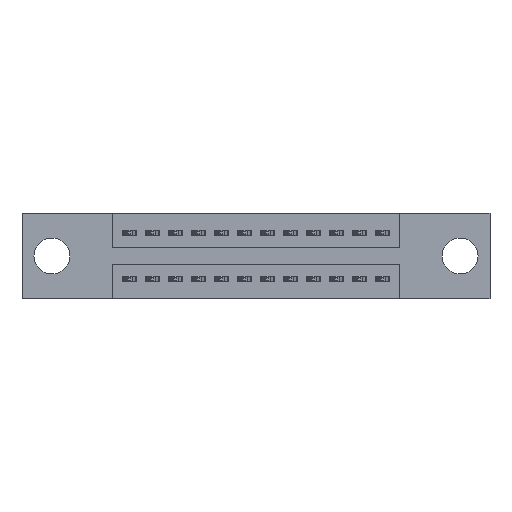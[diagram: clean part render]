
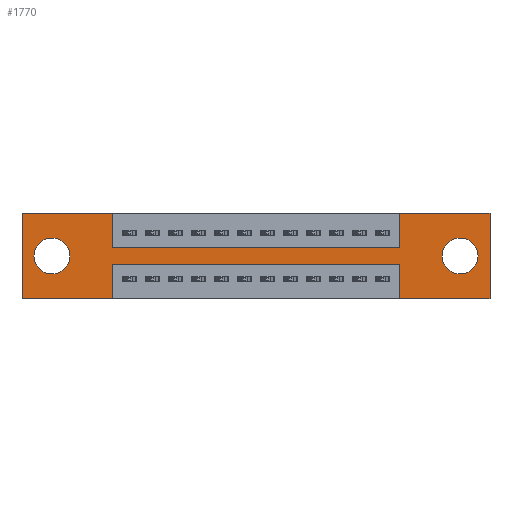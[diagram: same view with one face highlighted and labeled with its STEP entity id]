
A CAD part, front view. The second image highlights one B-rep face of the part: STEP entity #1770.
In plain terms, the highlighted planar face has unit normal (0, -1, 0).
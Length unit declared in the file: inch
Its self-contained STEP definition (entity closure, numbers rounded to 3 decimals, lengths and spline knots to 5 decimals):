
#2 = DIRECTION ( 'NONE',  ( 0., 0., -1. ) ) ;
#174 = DIRECTION ( 'NONE',  ( 0., -1., 0. ) ) ;
#203 = DIRECTION ( 'NONE',  ( 0., 0., -1. ) ) ;
#253 = CARTESIAN_POINT ( 'NONE',  ( 1.905, 0., -0.185 ) ) ;
#275 = LINE ( 'NONE', #10643, #8796 ) ;
#563 = DIRECTION ( 'NONE',  ( 0., 0., -1. ) ) ;
#569 = DIRECTION ( 'NONE',  ( 1., 0., 0. ) ) ;
#719 = VERTEX_POINT ( 'NONE', #10996 ) ;
#798 = CIRCLE ( 'NONE', #2338, 0.078 ) ;
#893 = EDGE_CURVE ( 'NONE', #12696, #719, #12292, .T. ) ;
#922 = VECTOR ( 'NONE', #13140, 39.37008 ) ;
#1003 = ORIENTED_EDGE ( 'NONE', *, *, #2645, .F. ) ;
#1030 = ORIENTED_EDGE ( 'NONE', *, *, #3036, .F. ) ;
#1304 = EDGE_CURVE ( 'NONE', #5290, #9071, #12277, .T. ) ;
#1329 = EDGE_LOOP ( 'NONE', ( #4029, #4434 ) ) ;
#1459 = DIRECTION ( 'NONE',  ( 0., 0., -1. ) ) ;
#1677 = CARTESIAN_POINT ( 'NONE',  ( 0., 0., -0.37 ) ) ;
#1770 = ADVANCED_FACE ( 'NONE', ( #9469, #12102, #7418 ), #4141, .T. ) ;
#1954 = DIRECTION ( 'NONE',  ( 1., 0., 0. ) ) ;
#2064 = ORIENTED_EDGE ( 'NONE', *, *, #10135, .F. ) ;
#2110 = CARTESIAN_POINT ( 'NONE',  ( 0.13, 0., -0.263 ) ) ;
#2338 = AXIS2_PLACEMENT_3D ( 'NONE', #253, #7798, #1459 ) ;
#2645 = EDGE_CURVE ( 'NONE', #11513, #3773, #12827, .T. ) ;
#2781 = LINE ( 'NONE', #10382, #10631 ) ;
#2795 = VECTOR ( 'NONE', #8695, 39.37008 ) ;
#2805 = VERTEX_POINT ( 'NONE', #12296 ) ;
#2915 = VECTOR ( 'NONE', #6998, 39.37008 ) ;
#3036 = EDGE_CURVE ( 'NONE', #3773, #12247, #275, .T. ) ;
#3151 = CARTESIAN_POINT ( 'NONE',  ( 0.3925, 0., -0.15 ) ) ;
#3304 = LINE ( 'NONE', #12684, #8466 ) ;
#3378 = ORIENTED_EDGE ( 'NONE', *, *, #8499, .T. ) ;
#3497 = CARTESIAN_POINT ( 'NONE',  ( 2.035, 0., 0. ) ) ;
#3583 = AXIS2_PLACEMENT_3D ( 'NONE', #12540, #6571, #2 ) ;
#3650 = ORIENTED_EDGE ( 'NONE', *, *, #12038, .F. ) ;
#3750 = VERTEX_POINT ( 'NONE', #4860 ) ;
#3773 = VERTEX_POINT ( 'NONE', #4777 ) ;
#3860 = ORIENTED_EDGE ( 'NONE', *, *, #7629, .T. ) ;
#3925 = EDGE_LOOP ( 'NONE', ( #6591, #10969, #7562, #7850, #9194, #2064, #1030, #1003, #3650, #5429, #10822, #8170 ) ) ;
#4004 = CARTESIAN_POINT ( 'NONE',  ( 2.035, 0., 0. ) ) ;
#4029 = ORIENTED_EDGE ( 'NONE', *, *, #4205, .T. ) ;
#4141 = PLANE ( 'NONE',  #5657 ) ;
#4205 = EDGE_CURVE ( 'NONE', #9071, #5290, #13422, .T. ) ;
#4434 = ORIENTED_EDGE ( 'NONE', *, *, #1304, .T. ) ;
#4455 = CARTESIAN_POINT ( 'NONE',  ( 0.3925, 0., -0.22 ) ) ;
#4621 = EDGE_CURVE ( 'NONE', #719, #4875, #3304, .T. ) ;
#4636 = VERTEX_POINT ( 'NONE', #11166 ) ;
#4777 = CARTESIAN_POINT ( 'NONE',  ( 1.6425, 0., -0.15 ) ) ;
#4835 = DIRECTION ( 'NONE',  ( 0., 1., 0. ) ) ;
#4860 = CARTESIAN_POINT ( 'NONE',  ( 0., 0., -0.37 ) ) ;
#4875 = VERTEX_POINT ( 'NONE', #5121 ) ;
#5099 = CARTESIAN_POINT ( 'NONE',  ( 1.905, 0., -0.263 ) ) ;
#5121 = CARTESIAN_POINT ( 'NONE',  ( 1.6425, 0., -0.22 ) ) ;
#5290 = VERTEX_POINT ( 'NONE', #2110 ) ;
#5429 = ORIENTED_EDGE ( 'NONE', *, *, #13178, .F. ) ;
#5558 = VECTOR ( 'NONE', #6076, 39.37008 ) ;
#5657 = AXIS2_PLACEMENT_3D ( 'NONE', #11202, #174, #203 ) ;
#5718 = LINE ( 'NONE', #11992, #2915 ) ;
#5762 = VERTEX_POINT ( 'NONE', #5099 ) ;
#5989 = DIRECTION ( 'NONE',  ( -1., 0., 0. ) ) ;
#6076 = DIRECTION ( 'NONE',  ( 0., 0., -1. ) ) ;
#6476 = CARTESIAN_POINT ( 'NONE',  ( 2.035, 0., -0.37 ) ) ;
#6571 = DIRECTION ( 'NONE',  ( 0., 1., 0. ) ) ;
#6591 = ORIENTED_EDGE ( 'NONE', *, *, #11502, .F. ) ;
#6746 = EDGE_LOOP ( 'NONE', ( #3378, #3860 ) ) ;
#6996 = VECTOR ( 'NONE', #569, 39.37008 ) ;
#6998 = DIRECTION ( 'NONE',  ( 1., 0., 0. ) ) ;
#7048 = DIRECTION ( 'NONE',  ( 0., 0., 1. ) ) ;
#7371 = AXIS2_PLACEMENT_3D ( 'NONE', #11588, #10906, #10991 ) ;
#7418 = FACE_OUTER_BOUND ( 'NONE', #3925, .T. ) ;
#7511 = CARTESIAN_POINT ( 'NONE',  ( 0.13, 0., -0.107 ) ) ;
#7540 = VECTOR ( 'NONE', #1954, 39.37008 ) ;
#7562 = ORIENTED_EDGE ( 'NONE', *, *, #4621, .F. ) ;
#7629 = EDGE_CURVE ( 'NONE', #5762, #2805, #8946, .T. ) ;
#7676 = CARTESIAN_POINT ( 'NONE',  ( 0.3925, 0., 0. ) ) ;
#7798 = DIRECTION ( 'NONE',  ( 0., 1., 0. ) ) ;
#7807 = VERTEX_POINT ( 'NONE', #9737 ) ;
#7850 = ORIENTED_EDGE ( 'NONE', *, *, #893, .F. ) ;
#7951 = EDGE_CURVE ( 'NONE', #7807, #3750, #12496, .T. ) ;
#8170 = ORIENTED_EDGE ( 'NONE', *, *, #7951, .F. ) ;
#8466 = VECTOR ( 'NONE', #11372, 39.37008 ) ;
#8499 = EDGE_CURVE ( 'NONE', #2805, #5762, #798, .T. ) ;
#8695 = DIRECTION ( 'NONE',  ( 0., 0., -1. ) ) ;
#8796 = VECTOR ( 'NONE', #10608, 39.37008 ) ;
#8946 = CIRCLE ( 'NONE', #3583, 0.078 ) ;
#9071 = VERTEX_POINT ( 'NONE', #7511 ) ;
#9084 = EDGE_CURVE ( 'NONE', #4875, #12977, #12925, .T. ) ;
#9194 = ORIENTED_EDGE ( 'NONE', *, *, #10892, .F. ) ;
#9469 = FACE_BOUND ( 'NONE', #6746, .T. ) ;
#9737 = CARTESIAN_POINT ( 'NONE',  ( 0.3925, 0., -0.37 ) ) ;
#9957 = CARTESIAN_POINT ( 'NONE',  ( 1.6425, 0., 0. ) ) ;
#10007 = VECTOR ( 'NONE', #12520, 39.37008 ) ;
#10034 = AXIS2_PLACEMENT_3D ( 'NONE', #10175, #4835, #7048 ) ;
#10135 = EDGE_CURVE ( 'NONE', #12247, #12814, #5718, .T. ) ;
#10154 = CARTESIAN_POINT ( 'NONE',  ( 0., 0., -0.37 ) ) ;
#10175 = CARTESIAN_POINT ( 'NONE',  ( 0.13, 0., -0.185 ) ) ;
#10382 = CARTESIAN_POINT ( 'NONE',  ( 0., 0., 0. ) ) ;
#10608 = DIRECTION ( 'NONE',  ( 0., 0., 1. ) ) ;
#10631 = VECTOR ( 'NONE', #11397, 39.37008 ) ;
#10643 = CARTESIAN_POINT ( 'NONE',  ( 1.6425, 0., 0. ) ) ;
#10661 = VERTEX_POINT ( 'NONE', #12783 ) ;
#10822 = ORIENTED_EDGE ( 'NONE', *, *, #12610, .F. ) ;
#10891 = LINE ( 'NONE', #4004, #5558 ) ;
#10892 = EDGE_CURVE ( 'NONE', #12814, #12696, #10891, .T. ) ;
#10906 = DIRECTION ( 'NONE',  ( 0., 1., 0. ) ) ;
#10959 = LINE ( 'NONE', #7676, #2795 ) ;
#10969 = ORIENTED_EDGE ( 'NONE', *, *, #9084, .F. ) ;
#10991 = DIRECTION ( 'NONE',  ( 0., 0., 1. ) ) ;
#10996 = CARTESIAN_POINT ( 'NONE',  ( 1.6425, 0., -0.37 ) ) ;
#11166 = CARTESIAN_POINT ( 'NONE',  ( 0., 0., 0. ) ) ;
#11202 = CARTESIAN_POINT ( 'NONE',  ( 0., 0., -0.37 ) ) ;
#11292 = VECTOR ( 'NONE', #563, 39.37008 ) ;
#11372 = DIRECTION ( 'NONE',  ( 0., 0., 1. ) ) ;
#11397 = DIRECTION ( 'NONE',  ( 0., 0., 1. ) ) ;
#11502 = EDGE_CURVE ( 'NONE', #12977, #7807, #11597, .T. ) ;
#11513 = VERTEX_POINT ( 'NONE', #12044 ) ;
#11588 = CARTESIAN_POINT ( 'NONE',  ( 0.13, 0., -0.185 ) ) ;
#11597 = LINE ( 'NONE', #12981, #11292 ) ;
#11847 = CARTESIAN_POINT ( 'NONE',  ( 0.3925, 0., -0.22 ) ) ;
#11992 = CARTESIAN_POINT ( 'NONE',  ( 0., 0., 0. ) ) ;
#12038 = EDGE_CURVE ( 'NONE', #10661, #11513, #10959, .T. ) ;
#12044 = CARTESIAN_POINT ( 'NONE',  ( 0.3925, 0., -0.15 ) ) ;
#12055 = CARTESIAN_POINT ( 'NONE',  ( 0., 0., 0. ) ) ;
#12102 = FACE_BOUND ( 'NONE', #1329, .T. ) ;
#12191 = VECTOR ( 'NONE', #5989, 39.37008 ) ;
#12247 = VERTEX_POINT ( 'NONE', #9957 ) ;
#12277 = CIRCLE ( 'NONE', #10034, 0.078 ) ;
#12292 = LINE ( 'NONE', #10154, #922 ) ;
#12296 = CARTESIAN_POINT ( 'NONE',  ( 1.905, 0., -0.107 ) ) ;
#12496 = LINE ( 'NONE', #1677, #12191 ) ;
#12520 = DIRECTION ( 'NONE',  ( -1., 0., 0. ) ) ;
#12540 = CARTESIAN_POINT ( 'NONE',  ( 1.905, 0., -0.185 ) ) ;
#12610 = EDGE_CURVE ( 'NONE', #3750, #4636, #2781, .T. ) ;
#12615 = LINE ( 'NONE', #12055, #6996 ) ;
#12684 = CARTESIAN_POINT ( 'NONE',  ( 1.6425, 0., -0.37 ) ) ;
#12696 = VERTEX_POINT ( 'NONE', #6476 ) ;
#12783 = CARTESIAN_POINT ( 'NONE',  ( 0.3925, 0., 0. ) ) ;
#12814 = VERTEX_POINT ( 'NONE', #3497 ) ;
#12827 = LINE ( 'NONE', #3151, #7540 ) ;
#12925 = LINE ( 'NONE', #4455, #10007 ) ;
#12977 = VERTEX_POINT ( 'NONE', #11847 ) ;
#12981 = CARTESIAN_POINT ( 'NONE',  ( 0.3925, 0., -0.37 ) ) ;
#13140 = DIRECTION ( 'NONE',  ( -1., 0., 0. ) ) ;
#13178 = EDGE_CURVE ( 'NONE', #4636, #10661, #12615, .T. ) ;
#13422 = CIRCLE ( 'NONE', #7371, 0.078 ) ;
